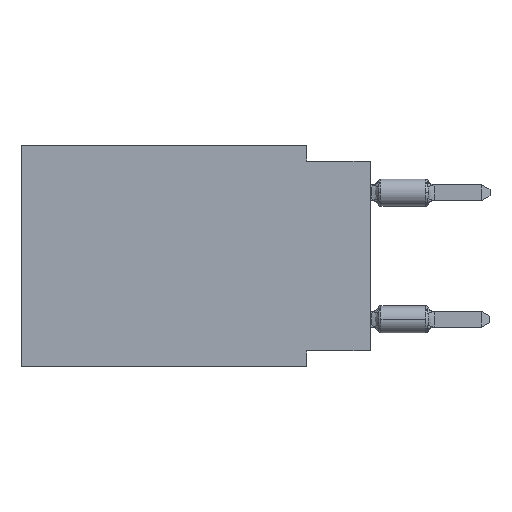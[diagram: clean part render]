
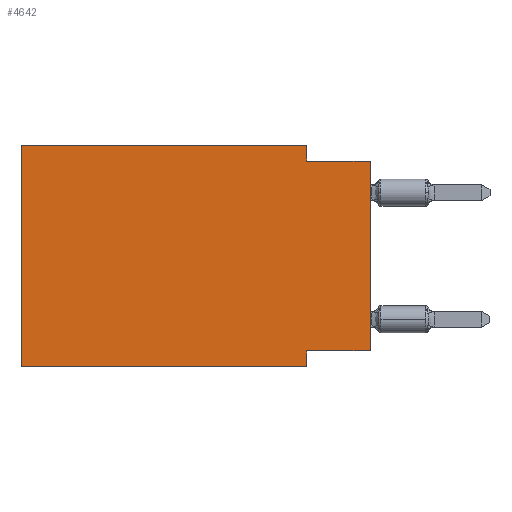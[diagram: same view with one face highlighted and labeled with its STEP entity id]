
A CAD part, left-side view. The second image highlights one B-rep face of the part: STEP entity #4642.
In plain terms, the highlighted planar face has unit normal (-1, 0, 0).
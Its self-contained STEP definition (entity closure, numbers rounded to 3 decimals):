
#362 = ORIENTED_EDGE ( 'NONE', *, *, #12628, .F. ) ;
#910 = VECTOR ( 'NONE', #10000, 1000. ) ;
#954 = EDGE_LOOP ( 'NONE', ( #8105, #11127, #362, #11378, #8671, #7137, #11409, #6203 ) ) ;
#1013 = LINE ( 'NONE', #13817, #1563 ) ;
#1051 = EDGE_CURVE ( 'NONE', #7116, #2442, #7884, .T. ) ;
#1563 = VECTOR ( 'NONE', #6306, 1000. ) ;
#1701 = LINE ( 'NONE', #1911, #4081 ) ;
#1851 = CARTESIAN_POINT ( 'NONE',  ( 0., 2.54, -8.89 ) ) ;
#1911 = CARTESIAN_POINT ( 'NONE',  ( 0., 0., -8.255 ) ) ;
#1931 = VERTEX_POINT ( 'NONE', #6076 ) ;
#1943 = VERTEX_POINT ( 'NONE', #1851 ) ;
#2123 = CARTESIAN_POINT ( 'NONE',  ( 0., 0., -8.255 ) ) ;
#2442 = VERTEX_POINT ( 'NONE', #10687 ) ;
#2918 = DIRECTION ( 'NONE',  ( 0., 0., -1. ) ) ;
#3363 = CARTESIAN_POINT ( 'NONE',  ( 0., 13.97, 0. ) ) ;
#3371 = VECTOR ( 'NONE', #9105, 1000. ) ;
#3394 = DIRECTION ( 'NONE',  ( 0., 0., 1. ) ) ;
#3572 = VECTOR ( 'NONE', #11100, 1000. ) ;
#3607 = CARTESIAN_POINT ( 'NONE',  ( 0., 0., -0.635 ) ) ;
#3684 = EDGE_CURVE ( 'NONE', #7116, #1931, #1701, .T. ) ;
#4081 = VECTOR ( 'NONE', #6141, 1000. ) ;
#4642 = ADVANCED_FACE ( 'NONE', ( #9309 ), #6371, .F. ) ;
#5766 = CARTESIAN_POINT ( 'NONE',  ( 0., 13.97, -8.89 ) ) ;
#5822 = VECTOR ( 'NONE', #2918, 1000. ) ;
#6076 = CARTESIAN_POINT ( 'NONE',  ( 0., 2.54, -8.255 ) ) ;
#6141 = DIRECTION ( 'NONE',  ( 0., 1., 0. ) ) ;
#6172 = LINE ( 'NONE', #13610, #7556 ) ;
#6203 = ORIENTED_EDGE ( 'NONE', *, *, #3684, .F. ) ;
#6306 = DIRECTION ( 'NONE',  ( 0., -1., 0. ) ) ;
#6371 = PLANE ( 'NONE',  #11481 ) ;
#6562 = CARTESIAN_POINT ( 'NONE',  ( 0., 0., 0. ) ) ;
#6857 = VERTEX_POINT ( 'NONE', #11316 ) ;
#6871 = CARTESIAN_POINT ( 'NONE',  ( 0., 2.54, 0. ) ) ;
#7116 = VERTEX_POINT ( 'NONE', #2123 ) ;
#7137 = ORIENTED_EDGE ( 'NONE', *, *, #9592, .T. ) ;
#7556 = VECTOR ( 'NONE', #11508, 1000. ) ;
#7884 = LINE ( 'NONE', #6562, #8953 ) ;
#8105 = ORIENTED_EDGE ( 'NONE', *, *, #1051, .T. ) ;
#8125 = LINE ( 'NONE', #8192, #5822 ) ;
#8192 = CARTESIAN_POINT ( 'NONE',  ( 0., 2.54, -8.89 ) ) ;
#8269 = LINE ( 'NONE', #6871, #3371 ) ;
#8360 = VERTEX_POINT ( 'NONE', #9199 ) ;
#8671 = ORIENTED_EDGE ( 'NONE', *, *, #9002, .F. ) ;
#8953 = VECTOR ( 'NONE', #3394, 1000. ) ;
#9002 = EDGE_CURVE ( 'NONE', #10883, #13641, #6172, .T. ) ;
#9105 = DIRECTION ( 'NONE',  ( 0., 0., -1. ) ) ;
#9131 = LINE ( 'NONE', #12163, #3572 ) ;
#9199 = CARTESIAN_POINT ( 'NONE',  ( 0., 2.54, 0. ) ) ;
#9309 = FACE_OUTER_BOUND ( 'NONE', #954, .T. ) ;
#9592 = EDGE_CURVE ( 'NONE', #10883, #1943, #9131, .T. ) ;
#10000 = DIRECTION ( 'NONE',  ( 0., -1., 0. ) ) ;
#10582 = EDGE_CURVE ( 'NONE', #1931, #1943, #8125, .T. ) ;
#10647 = DIRECTION ( 'NONE',  ( 1., 0., 0. ) ) ;
#10687 = CARTESIAN_POINT ( 'NONE',  ( 0., 0., -0.635 ) ) ;
#10883 = VERTEX_POINT ( 'NONE', #5766 ) ;
#11100 = DIRECTION ( 'NONE',  ( 0., -1., 0. ) ) ;
#11127 = ORIENTED_EDGE ( 'NONE', *, *, #13385, .F. ) ;
#11316 = CARTESIAN_POINT ( 'NONE',  ( 0., 2.54, -0.635 ) ) ;
#11378 = ORIENTED_EDGE ( 'NONE', *, *, #12670, .F. ) ;
#11409 = ORIENTED_EDGE ( 'NONE', *, *, #10582, .F. ) ;
#11481 = AXIS2_PLACEMENT_3D ( 'NONE', #13594, #10647, #12614 ) ;
#11508 = DIRECTION ( 'NONE',  ( 0., 0., 1. ) ) ;
#12163 = CARTESIAN_POINT ( 'NONE',  ( 0., 13.97, -8.89 ) ) ;
#12302 = LINE ( 'NONE', #3607, #910 ) ;
#12614 = DIRECTION ( 'NONE',  ( 0., 0., -1. ) ) ;
#12628 = EDGE_CURVE ( 'NONE', #8360, #6857, #8269, .T. ) ;
#12670 = EDGE_CURVE ( 'NONE', #13641, #8360, #1013, .T. ) ;
#13385 = EDGE_CURVE ( 'NONE', #6857, #2442, #12302, .T. ) ;
#13594 = CARTESIAN_POINT ( 'NONE',  ( 0., 13.97, 0. ) ) ;
#13610 = CARTESIAN_POINT ( 'NONE',  ( 0., 13.97, 0. ) ) ;
#13641 = VERTEX_POINT ( 'NONE', #3363 ) ;
#13817 = CARTESIAN_POINT ( 'NONE',  ( 0., 13.97, 0. ) ) ;
